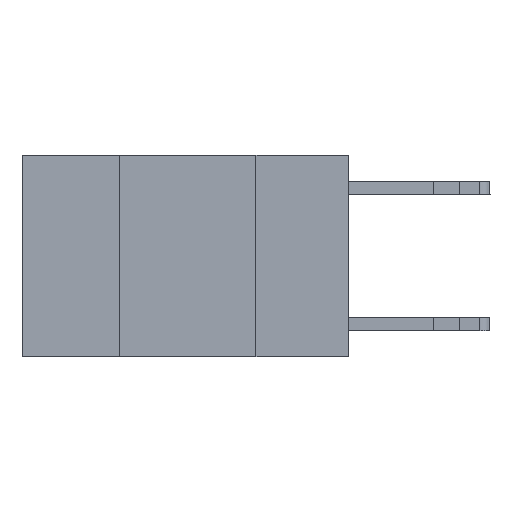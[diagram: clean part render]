
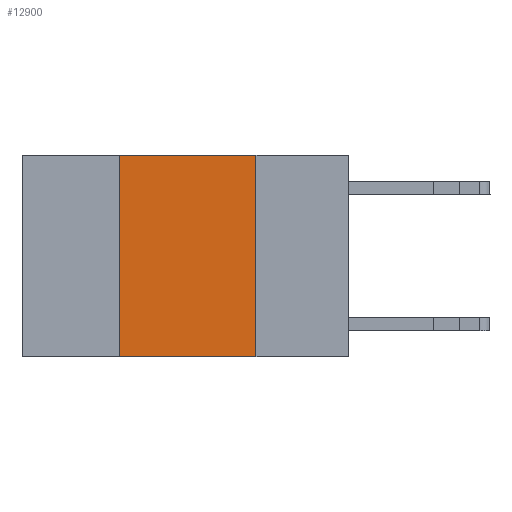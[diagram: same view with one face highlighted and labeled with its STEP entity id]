
A CAD part, left-side view. The second image highlights one B-rep face of the part: STEP entity #12900.
In plain terms, the highlighted planar face has unit normal (-1, 0, 0).
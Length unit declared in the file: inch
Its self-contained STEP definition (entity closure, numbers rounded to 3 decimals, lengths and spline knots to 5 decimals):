
#141 = CARTESIAN_POINT ( 'NONE',  ( 0., 0.17, 0. ) ) ;
#259 = EDGE_CURVE ( 'NONE', #11122, #2800, #14405, .T. ) ;
#793 = EDGE_CURVE ( 'NONE', #11122, #17385, #17055, .T. ) ;
#1342 = CARTESIAN_POINT ( 'NONE',  ( 0., 0.6, 0. ) ) ;
#2234 = ORIENTED_EDGE ( 'NONE', *, *, #7302, .F. ) ;
#2753 = DIRECTION ( 'NONE',  ( 1., 0., 0. ) ) ;
#2800 = VERTEX_POINT ( 'NONE', #7213 ) ;
#2897 = ORIENTED_EDGE ( 'NONE', *, *, #259, .T. ) ;
#3333 = ORIENTED_EDGE ( 'NONE', *, *, #793, .F. ) ;
#4639 = CARTESIAN_POINT ( 'NONE',  ( 0., 0.42, -0.37 ) ) ;
#6223 = AXIS2_PLACEMENT_3D ( 'NONE', #11017, #2753, #12390 ) ;
#6300 = LINE ( 'NONE', #141, #16655 ) ;
#7156 = VERTEX_POINT ( 'NONE', #17542 ) ;
#7213 = CARTESIAN_POINT ( 'NONE',  ( 0., 0.17, -0.37 ) ) ;
#7302 = EDGE_CURVE ( 'NONE', #7156, #2800, #6300, .T. ) ;
#7923 = VECTOR ( 'NONE', #11070, 39.37008 ) ;
#8820 = DIRECTION ( 'NONE',  ( 0., -1., 0. ) ) ;
#9305 = ORIENTED_EDGE ( 'NONE', *, *, #10575, .F. ) ;
#9791 = DIRECTION ( 'NONE',  ( 0., 0., -1. ) ) ;
#10229 = DIRECTION ( 'NONE',  ( 0., 0., 1. ) ) ;
#10282 = FACE_OUTER_BOUND ( 'NONE', #14830, .T. ) ;
#10575 = EDGE_CURVE ( 'NONE', #17385, #7156, #15148, .T. ) ;
#10714 = CARTESIAN_POINT ( 'NONE',  ( 0., 0.42, 0. ) ) ;
#10825 = VECTOR ( 'NONE', #8820, 39.37008 ) ;
#11017 = CARTESIAN_POINT ( 'NONE',  ( 0., 0.6, 0. ) ) ;
#11070 = DIRECTION ( 'NONE',  ( 0., -1., 0. ) ) ;
#11122 = VERTEX_POINT ( 'NONE', #4639 ) ;
#11535 = CARTESIAN_POINT ( 'NONE',  ( 0., 0.6, -0.37 ) ) ;
#12390 = DIRECTION ( 'NONE',  ( 0., 0., -1. ) ) ;
#12900 = ADVANCED_FACE ( 'NONE', ( #10282 ), #13675, .F. ) ;
#13675 = PLANE ( 'NONE',  #6223 ) ;
#13974 = CARTESIAN_POINT ( 'NONE',  ( 0., 0.42, 0. ) ) ;
#14405 = LINE ( 'NONE', #11535, #10825 ) ;
#14830 = EDGE_LOOP ( 'NONE', ( #2234, #9305, #3333, #2897 ) ) ;
#15148 = LINE ( 'NONE', #1342, #7923 ) ;
#16645 = VECTOR ( 'NONE', #10229, 39.37008 ) ;
#16655 = VECTOR ( 'NONE', #9791, 39.37008 ) ;
#17055 = LINE ( 'NONE', #13974, #16645 ) ;
#17385 = VERTEX_POINT ( 'NONE', #10714 ) ;
#17542 = CARTESIAN_POINT ( 'NONE',  ( 0., 0.17, 0. ) ) ;
